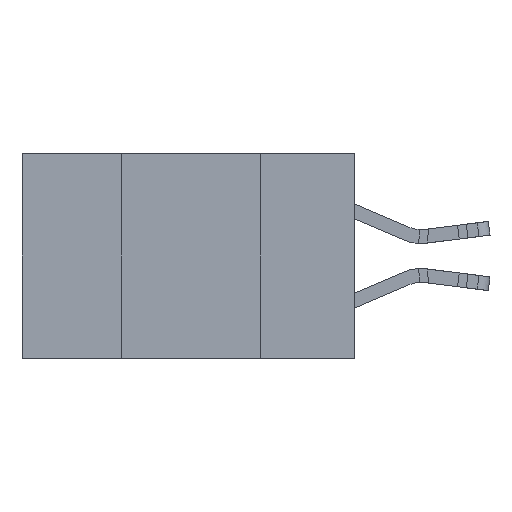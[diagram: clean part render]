
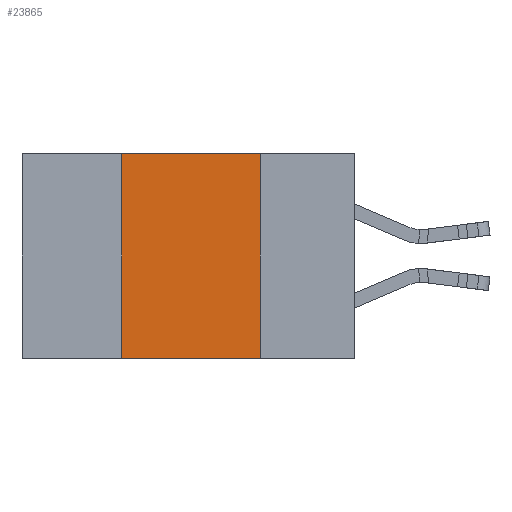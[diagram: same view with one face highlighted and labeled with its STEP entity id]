
A CAD part, left-side view. The second image highlights one B-rep face of the part: STEP entity #23865.
In plain terms, the highlighted planar face has unit normal (-1, 0, 0).
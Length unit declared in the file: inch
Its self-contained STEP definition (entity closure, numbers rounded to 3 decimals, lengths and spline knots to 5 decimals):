
#739 = AXIS2_PLACEMENT_3D ( 'NONE', #4193, #19995, #1682 ) ;
#887 = VERTEX_POINT ( 'NONE', #16012 ) ;
#1682 = DIRECTION ( 'NONE',  ( 0., 0., -1. ) ) ;
#1846 = LINE ( 'NONE', #3210, #5447 ) ;
#2234 = VERTEX_POINT ( 'NONE', #23877 ) ;
#3210 = CARTESIAN_POINT ( 'NONE',  ( 0., 0.42, 0. ) ) ;
#3688 = VECTOR ( 'NONE', #17015, 39.37008 ) ;
#4193 = CARTESIAN_POINT ( 'NONE',  ( 0., 0.6, 0. ) ) ;
#4663 = VERTEX_POINT ( 'NONE', #5448 ) ;
#4817 = FACE_OUTER_BOUND ( 'NONE', #20361, .T. ) ;
#5395 = LINE ( 'NONE', #19774, #6831 ) ;
#5447 = VECTOR ( 'NONE', #10127, 39.37008 ) ;
#5448 = CARTESIAN_POINT ( 'NONE',  ( 0., 0.17, 0. ) ) ;
#6293 = PLANE ( 'NONE',  #739 ) ;
#6831 = VECTOR ( 'NONE', #8392, 39.37008 ) ;
#8194 = ORIENTED_EDGE ( 'NONE', *, *, #21517, .F. ) ;
#8392 = DIRECTION ( 'NONE',  ( 0., 0., -1. ) ) ;
#10127 = DIRECTION ( 'NONE',  ( 0., 0., 1. ) ) ;
#10893 = VECTOR ( 'NONE', #11657, 39.37008 ) ;
#11657 = DIRECTION ( 'NONE',  ( 0., -1., 0. ) ) ;
#12359 = LINE ( 'NONE', #22829, #10893 ) ;
#15780 = EDGE_CURVE ( 'NONE', #18247, #887, #1846, .T. ) ;
#16012 = CARTESIAN_POINT ( 'NONE',  ( 0., 0.42, 0. ) ) ;
#17015 = DIRECTION ( 'NONE',  ( 0., -1., 0. ) ) ;
#18247 = VERTEX_POINT ( 'NONE', #20433 ) ;
#19774 = CARTESIAN_POINT ( 'NONE',  ( 0., 0.17, 0. ) ) ;
#19916 = ORIENTED_EDGE ( 'NONE', *, *, #15780, .F. ) ;
#19995 = DIRECTION ( 'NONE',  ( 1., 0., 0. ) ) ;
#20361 = EDGE_LOOP ( 'NONE', ( #29026, #8194, #19916, #20738 ) ) ;
#20433 = CARTESIAN_POINT ( 'NONE',  ( 0., 0.42, -0.37 ) ) ;
#20738 = ORIENTED_EDGE ( 'NONE', *, *, #24707, .T. ) ;
#21517 = EDGE_CURVE ( 'NONE', #887, #4663, #23835, .T. ) ;
#22315 = EDGE_CURVE ( 'NONE', #4663, #2234, #5395, .T. ) ;
#22829 = CARTESIAN_POINT ( 'NONE',  ( 0., 0.6, -0.37 ) ) ;
#23835 = LINE ( 'NONE', #24151, #3688 ) ;
#23865 = ADVANCED_FACE ( 'NONE', ( #4817 ), #6293, .F. ) ;
#23877 = CARTESIAN_POINT ( 'NONE',  ( 0., 0.17, -0.37 ) ) ;
#24151 = CARTESIAN_POINT ( 'NONE',  ( 0., 0.6, 0. ) ) ;
#24707 = EDGE_CURVE ( 'NONE', #18247, #2234, #12359, .T. ) ;
#29026 = ORIENTED_EDGE ( 'NONE', *, *, #22315, .F. ) ;
